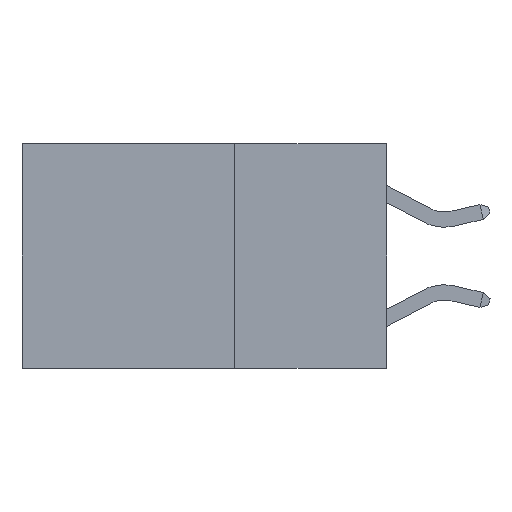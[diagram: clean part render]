
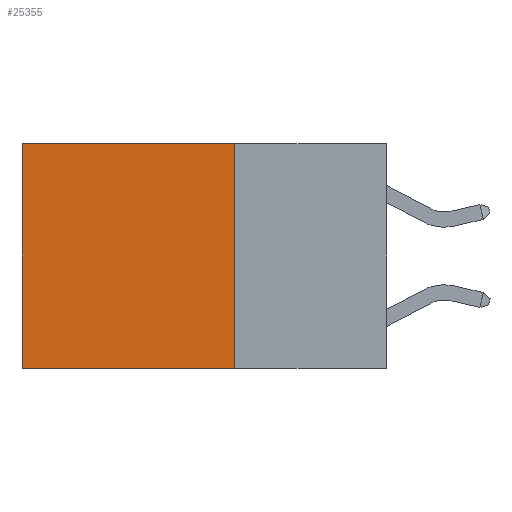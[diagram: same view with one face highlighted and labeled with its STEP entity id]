
A CAD part, left-side view. The second image highlights one B-rep face of the part: STEP entity #25355.
In plain terms, the highlighted planar face has unit normal (-1, 0, 0).
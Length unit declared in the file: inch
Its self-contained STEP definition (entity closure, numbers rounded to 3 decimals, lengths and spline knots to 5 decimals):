
#60 = FACE_OUTER_BOUND ( 'NONE', #26958, .T. ) ;
#192 = DIRECTION ( 'NONE',  ( 0., 0., -1. ) ) ;
#389 = EDGE_CURVE ( 'NONE', #14578, #28447, #15977, .T. ) ;
#1163 = DIRECTION ( 'NONE',  ( 0., 0., -1. ) ) ;
#2380 = CARTESIAN_POINT ( 'NONE',  ( 0.2625, 0.25, 0. ) ) ;
#2808 = AXIS2_PLACEMENT_3D ( 'NONE', #20485, #15704, #1163 ) ;
#4812 = VERTEX_POINT ( 'NONE', #6841 ) ;
#6841 = CARTESIAN_POINT ( 'NONE',  ( 0.2625, 0.6, 0. ) ) ;
#7228 = EDGE_CURVE ( 'NONE', #4812, #11734, #22000, .T. ) ;
#9207 = ORIENTED_EDGE ( 'NONE', *, *, #13408, .T. ) ;
#9952 = CARTESIAN_POINT ( 'NONE',  ( 0.2625, 0.25, -0.37 ) ) ;
#11734 = VERTEX_POINT ( 'NONE', #18917 ) ;
#13165 = LINE ( 'NONE', #9952, #18858 ) ;
#13263 = PLANE ( 'NONE',  #2808 ) ;
#13408 = EDGE_CURVE ( 'NONE', #14578, #4812, #23828, .T. ) ;
#14240 = EDGE_CURVE ( 'NONE', #28447, #11734, #13165, .T. ) ;
#14578 = VERTEX_POINT ( 'NONE', #18499 ) ;
#15704 = DIRECTION ( 'NONE',  ( 1., 0., 0. ) ) ;
#15977 = LINE ( 'NONE', #2380, #20134 ) ;
#16565 = ORIENTED_EDGE ( 'NONE', *, *, #389, .F. ) ;
#17405 = VECTOR ( 'NONE', #17460, 39.37008 ) ;
#17460 = DIRECTION ( 'NONE',  ( 0., 1., 0. ) ) ;
#18499 = CARTESIAN_POINT ( 'NONE',  ( 0.2625, 0.25, 0. ) ) ;
#18858 = VECTOR ( 'NONE', #24430, 39.37008 ) ;
#18917 = CARTESIAN_POINT ( 'NONE',  ( 0.2625, 0.6, -0.37 ) ) ;
#20134 = VECTOR ( 'NONE', #192, 39.37008 ) ;
#20485 = CARTESIAN_POINT ( 'NONE',  ( 0.2625, 0.25, 0. ) ) ;
#22000 = LINE ( 'NONE', #22824, #27622 ) ;
#22673 = ORIENTED_EDGE ( 'NONE', *, *, #7228, .T. ) ;
#22824 = CARTESIAN_POINT ( 'NONE',  ( 0.2625, 0.6, 0. ) ) ;
#23828 = LINE ( 'NONE', #29442, #17405 ) ;
#23973 = CARTESIAN_POINT ( 'NONE',  ( 0.2625, 0.25, -0.37 ) ) ;
#24430 = DIRECTION ( 'NONE',  ( 0., 1., 0. ) ) ;
#25213 = DIRECTION ( 'NONE',  ( 0., 0., -1. ) ) ;
#25355 = ADVANCED_FACE ( 'NONE', ( #60 ), #13263, .F. ) ;
#26958 = EDGE_LOOP ( 'NONE', ( #22673, #31093, #16565, #9207 ) ) ;
#27622 = VECTOR ( 'NONE', #25213, 39.37008 ) ;
#28447 = VERTEX_POINT ( 'NONE', #23973 ) ;
#29442 = CARTESIAN_POINT ( 'NONE',  ( 0.2625, 0.25, 0. ) ) ;
#31093 = ORIENTED_EDGE ( 'NONE', *, *, #14240, .F. ) ;
